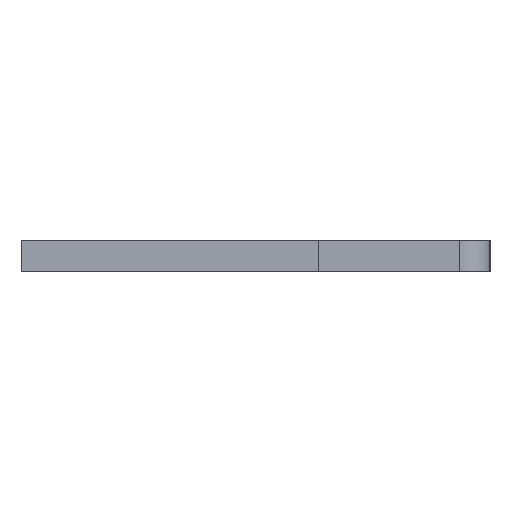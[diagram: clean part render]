
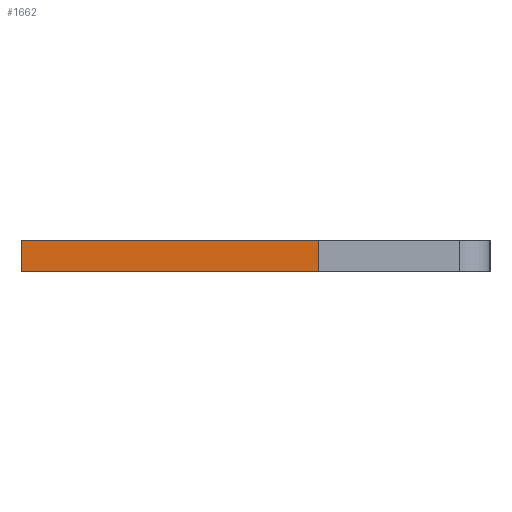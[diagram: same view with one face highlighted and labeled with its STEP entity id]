
A CAD part, left-side view. The second image highlights one B-rep face of the part: STEP entity #1662.
In plain terms, the highlighted face is planar.
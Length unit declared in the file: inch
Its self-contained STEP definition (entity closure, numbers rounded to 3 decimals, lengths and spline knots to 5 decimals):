
#78 = EDGE_CURVE ( 'NONE', #1343, #922, #1364, .T. ) ;
#114 = EDGE_CURVE ( 'NONE', #235, #1343, #1810, .T. ) ;
#188 = DIRECTION ( 'NONE',  ( 0., 1., 0. ) ) ;
#222 = ORIENTED_EDGE ( 'NONE', *, *, #78, .T. ) ;
#235 = VERTEX_POINT ( 'NONE', #1598 ) ;
#250 = PLANE ( 'NONE',  #832 ) ;
#262 = ORIENTED_EDGE ( 'NONE', *, *, #699, .F. ) ;
#342 = CARTESIAN_POINT ( 'NONE',  ( 0.01, 0.15, -0.04 ) ) ;
#534 = CARTESIAN_POINT ( 'NONE',  ( 0.01, 0.15, -0.04 ) ) ;
#574 = VECTOR ( 'NONE', #604, 39.37008 ) ;
#594 = DIRECTION ( 'NONE',  ( 1., 0., 0. ) ) ;
#604 = DIRECTION ( 'NONE',  ( -1., 0., 0. ) ) ;
#636 = FACE_OUTER_BOUND ( 'NONE', #1012, .T. ) ;
#682 = VECTOR ( 'NONE', #759, 39.37008 ) ;
#699 = EDGE_CURVE ( 'NONE', #235, #838, #1793, .T. ) ;
#759 = DIRECTION ( 'NONE',  ( 0., 1., 0. ) ) ;
#780 = ORIENTED_EDGE ( 'NONE', *, *, #1984, .F. ) ;
#832 = AXIS2_PLACEMENT_3D ( 'NONE', #1101, #1760, #594 ) ;
#838 = VERTEX_POINT ( 'NONE', #342 ) ;
#922 = VERTEX_POINT ( 'NONE', #1900 ) ;
#1012 = EDGE_LOOP ( 'NONE', ( #222, #780, #262, #1508 ) ) ;
#1019 = DIRECTION ( 'NONE',  ( -1., 0., 0. ) ) ;
#1101 = CARTESIAN_POINT ( 'NONE',  ( 0.01, 0.15, -0.04 ) ) ;
#1336 = LINE ( 'NONE', #534, #1812 ) ;
#1343 = VERTEX_POINT ( 'NONE', #1720 ) ;
#1359 = CARTESIAN_POINT ( 'NONE',  ( 0.01, 0.15, -0.04 ) ) ;
#1364 = LINE ( 'NONE', #1608, #682 ) ;
#1508 = ORIENTED_EDGE ( 'NONE', *, *, #114, .T. ) ;
#1591 = CARTESIAN_POINT ( 'NONE',  ( 0.01, -0.04, -0.04 ) ) ;
#1598 = CARTESIAN_POINT ( 'NONE',  ( 0.01, -0.04, -0.04 ) ) ;
#1608 = CARTESIAN_POINT ( 'NONE',  ( -0.01, 0.15, -0.04 ) ) ;
#1662 = ADVANCED_FACE ( 'NONE', ( #636 ), #250, .F. ) ;
#1712 = VECTOR ( 'NONE', #188, 39.37008 ) ;
#1720 = CARTESIAN_POINT ( 'NONE',  ( -0.01, -0.04, -0.04 ) ) ;
#1760 = DIRECTION ( 'NONE',  ( 0., 0., 1. ) ) ;
#1793 = LINE ( 'NONE', #1359, #1712 ) ;
#1810 = LINE ( 'NONE', #1591, #574 ) ;
#1812 = VECTOR ( 'NONE', #1019, 39.37008 ) ;
#1900 = CARTESIAN_POINT ( 'NONE',  ( -0.01, 0.15, -0.04 ) ) ;
#1984 = EDGE_CURVE ( 'NONE', #838, #922, #1336, .T. ) ;
